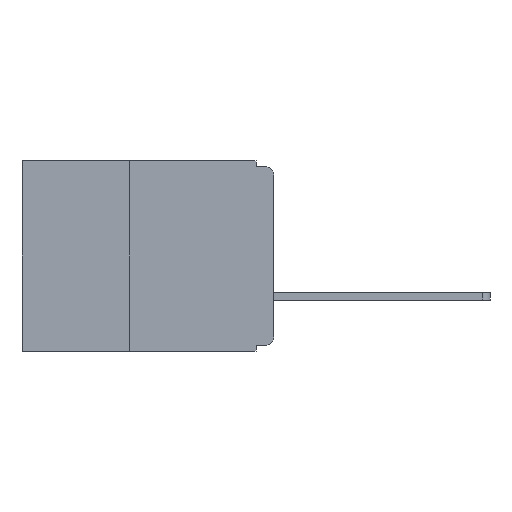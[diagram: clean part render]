
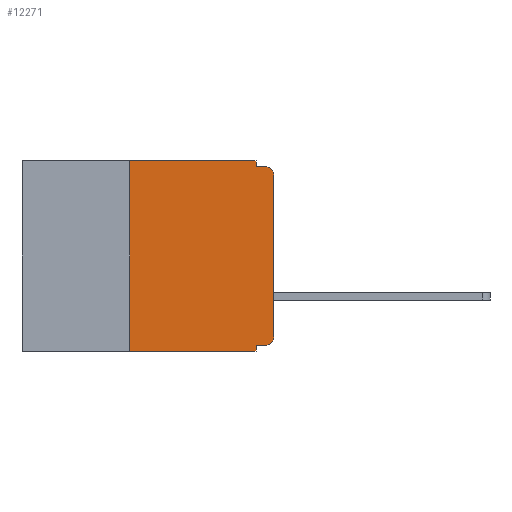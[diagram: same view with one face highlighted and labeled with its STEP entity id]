
A CAD part, left-side view. The second image highlights one B-rep face of the part: STEP entity #12271.
In plain terms, the highlighted planar face has unit normal (-1, 0, 0).
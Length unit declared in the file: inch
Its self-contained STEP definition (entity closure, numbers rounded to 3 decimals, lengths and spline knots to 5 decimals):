
#369 = VERTEX_POINT ( 'NONE', #20853 ) ;
#658 = EDGE_CURVE ( 'NONE', #7189, #5975, #6311, .T. ) ;
#802 = LINE ( 'NONE', #5387, #4933 ) ;
#1218 = CARTESIAN_POINT ( 'NONE',  ( 0., 0.015, -0.01 ) ) ;
#1596 = CARTESIAN_POINT ( 'NONE',  ( 0., 0., -0.01 ) ) ;
#2017 = LINE ( 'NONE', #11123, #19359 ) ;
#2104 = PLANE ( 'NONE',  #12999 ) ;
#2177 = CARTESIAN_POINT ( 'NONE',  ( 0., 0.031, -0.32 ) ) ;
#2723 = CARTESIAN_POINT ( 'NONE',  ( 0., 0.031, -0.33 ) ) ;
#3179 = VECTOR ( 'NONE', #13688, 39.37008 ) ;
#3546 = DIRECTION ( 'NONE',  ( 0., 0., -1. ) ) ;
#3741 = LINE ( 'NONE', #8530, #3179 ) ;
#3831 = EDGE_LOOP ( 'NONE', ( #9036, #10067, #10210, #10786, #11089, #11731, #12545, #12571, #12738, #13137 ) ) ;
#4405 = DIRECTION ( 'NONE',  ( 0., -1., 0. ) ) ;
#4740 = CARTESIAN_POINT ( 'NONE',  ( 0., 0.015, -0.32 ) ) ;
#4933 = VECTOR ( 'NONE', #14103, 39.37008 ) ;
#4976 = AXIS2_PLACEMENT_3D ( 'NONE', #20301, #10434, #3546 ) ;
#5222 = DIRECTION ( 'NONE',  ( -1., 0., 0. ) ) ;
#5387 = CARTESIAN_POINT ( 'NONE',  ( 0., 0.031, 0. ) ) ;
#5856 = CARTESIAN_POINT ( 'NONE',  ( 0., 0.031, -0.33 ) ) ;
#5975 = VERTEX_POINT ( 'NONE', #1218 ) ;
#6194 = DIRECTION ( 'NONE',  ( 0., 0., -1. ) ) ;
#6311 = CIRCLE ( 'NONE', #4976, 0.015 ) ;
#6402 = VERTEX_POINT ( 'NONE', #5856 ) ;
#6820 = EDGE_CURVE ( 'NONE', #21253, #9592, #802, .T. ) ;
#7189 = VERTEX_POINT ( 'NONE', #20260 ) ;
#7282 = CARTESIAN_POINT ( 'NONE',  ( 0., 0.031, -0.01 ) ) ;
#7329 = DIRECTION ( 'NONE',  ( 1., 0., 0. ) ) ;
#7386 = CARTESIAN_POINT ( 'NONE',  ( 0., 0.031, 0. ) ) ;
#7934 = CARTESIAN_POINT ( 'NONE',  ( 0., 0.25, -0.33 ) ) ;
#8002 = LINE ( 'NONE', #18245, #21245 ) ;
#8228 = FACE_OUTER_BOUND ( 'NONE', #3831, .T. ) ;
#8530 = CARTESIAN_POINT ( 'NONE',  ( 0., 0.25, -0.33 ) ) ;
#9036 = ORIENTED_EDGE ( 'NONE', *, *, #10321, .T. ) ;
#9592 = VERTEX_POINT ( 'NONE', #7282 ) ;
#9835 = VERTEX_POINT ( 'NONE', #7934 ) ;
#9856 = EDGE_CURVE ( 'NONE', #369, #21253, #20972, .T. ) ;
#10067 = ORIENTED_EDGE ( 'NONE', *, *, #658, .T. ) ;
#10210 = ORIENTED_EDGE ( 'NONE', *, *, #14800, .F. ) ;
#10321 = EDGE_CURVE ( 'NONE', #22104, #7189, #2017, .T. ) ;
#10434 = DIRECTION ( 'NONE',  ( -1., 0., 0. ) ) ;
#10786 = ORIENTED_EDGE ( 'NONE', *, *, #6820, .F. ) ;
#11089 = ORIENTED_EDGE ( 'NONE', *, *, #9856, .F. ) ;
#11123 = CARTESIAN_POINT ( 'NONE',  ( 0., 0., 0. ) ) ;
#11508 = CARTESIAN_POINT ( 'NONE',  ( 0., 0., -0.32 ) ) ;
#11520 = CARTESIAN_POINT ( 'NONE',  ( 0., 0.437, 0. ) ) ;
#11731 = ORIENTED_EDGE ( 'NONE', *, *, #15953, .F. ) ;
#12131 = LINE ( 'NONE', #11508, #16200 ) ;
#12271 = ADVANCED_FACE ( 'NONE', ( #8228 ), #2104, .F. ) ;
#12303 = VERTEX_POINT ( 'NONE', #2177 ) ;
#12493 = CARTESIAN_POINT ( 'NONE',  ( 0., 0.437, 0. ) ) ;
#12545 = ORIENTED_EDGE ( 'NONE', *, *, #20777, .T. ) ;
#12571 = ORIENTED_EDGE ( 'NONE', *, *, #13912, .F. ) ;
#12738 = ORIENTED_EDGE ( 'NONE', *, *, #15751, .F. ) ;
#12864 = DIRECTION ( 'NONE',  ( 0., 0., 1. ) ) ;
#12999 = AXIS2_PLACEMENT_3D ( 'NONE', #12493, #7329, #19449 ) ;
#13137 = ORIENTED_EDGE ( 'NONE', *, *, #21070, .T. ) ;
#13257 = DIRECTION ( 'NONE',  ( 0., 1., 0. ) ) ;
#13688 = DIRECTION ( 'NONE',  ( 0., 0., 1. ) ) ;
#13729 = DIRECTION ( 'NONE',  ( 0., -1., 0. ) ) ;
#13847 = VECTOR ( 'NONE', #6194, 39.37008 ) ;
#13912 = EDGE_CURVE ( 'NONE', #12303, #6402, #18451, .T. ) ;
#14103 = DIRECTION ( 'NONE',  ( 0., 0., -1. ) ) ;
#14800 = EDGE_CURVE ( 'NONE', #9592, #5975, #18945, .T. ) ;
#15579 = CARTESIAN_POINT ( 'NONE',  ( 0., 0.015, -0.305 ) ) ;
#15751 = EDGE_CURVE ( 'NONE', #18766, #12303, #12131, .T. ) ;
#15876 = VECTOR ( 'NONE', #21815, 39.37008 ) ;
#15877 = AXIS2_PLACEMENT_3D ( 'NONE', #15579, #5222, #17340 ) ;
#15879 = CIRCLE ( 'NONE', #15877, 0.015 ) ;
#15953 = EDGE_CURVE ( 'NONE', #9835, #369, #3741, .T. ) ;
#16200 = VECTOR ( 'NONE', #13257, 39.37008 ) ;
#17340 = DIRECTION ( 'NONE',  ( 0., 0., -1. ) ) ;
#18245 = CARTESIAN_POINT ( 'NONE',  ( 0., 0.437, -0.33 ) ) ;
#18451 = LINE ( 'NONE', #2723, #13847 ) ;
#18766 = VERTEX_POINT ( 'NONE', #4740 ) ;
#18945 = LINE ( 'NONE', #1596, #22402 ) ;
#19359 = VECTOR ( 'NONE', #12864, 39.37008 ) ;
#19449 = DIRECTION ( 'NONE',  ( 0., 0., -1. ) ) ;
#20260 = CARTESIAN_POINT ( 'NONE',  ( 0., 0., -0.025 ) ) ;
#20301 = CARTESIAN_POINT ( 'NONE',  ( 0., 0.015, -0.025 ) ) ;
#20433 = CARTESIAN_POINT ( 'NONE',  ( 0., 0., -0.305 ) ) ;
#20777 = EDGE_CURVE ( 'NONE', #9835, #6402, #8002, .T. ) ;
#20853 = CARTESIAN_POINT ( 'NONE',  ( 0., 0.25, 0. ) ) ;
#20972 = LINE ( 'NONE', #11520, #15876 ) ;
#21070 = EDGE_CURVE ( 'NONE', #18766, #22104, #15879, .T. ) ;
#21245 = VECTOR ( 'NONE', #4405, 39.37008 ) ;
#21253 = VERTEX_POINT ( 'NONE', #7386 ) ;
#21815 = DIRECTION ( 'NONE',  ( 0., -1., 0. ) ) ;
#22104 = VERTEX_POINT ( 'NONE', #20433 ) ;
#22402 = VECTOR ( 'NONE', #13729, 39.37008 ) ;
